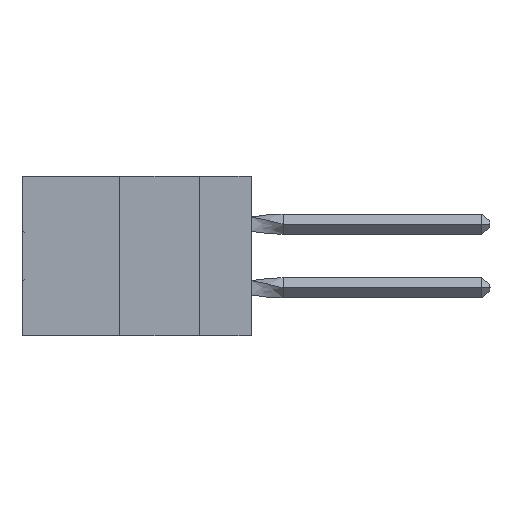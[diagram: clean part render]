
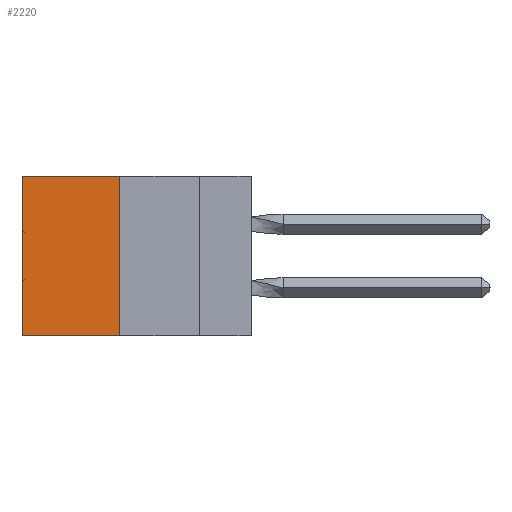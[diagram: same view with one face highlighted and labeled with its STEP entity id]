
A CAD part, left-side view. The second image highlights one B-rep face of the part: STEP entity #2220.
In plain terms, the highlighted planar face has unit normal (-1, 0, 0).
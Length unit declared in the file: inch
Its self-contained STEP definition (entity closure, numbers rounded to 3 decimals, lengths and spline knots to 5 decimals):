
#1751 = ORIENTED_EDGE ( 'NONE', *, *, #40516, .F. ) ;
#1928 = ORIENTED_EDGE ( 'NONE', *, *, #43611, .T. ) ;
#2220 = ADVANCED_FACE ( 'NONE', ( #25682 ), #41466, .F. ) ;
#5457 = LINE ( 'NONE', #10869, #13340 ) ;
#10869 = CARTESIAN_POINT ( 'NONE',  ( 0.305, 0.413, -0.5 ) ) ;
#13340 = VECTOR ( 'NONE', #15083, 39.37008 ) ;
#15083 = DIRECTION ( 'NONE',  ( 0., 1., 0. ) ) ;
#15513 = LINE ( 'NONE', #37387, #19696 ) ;
#15803 = VECTOR ( 'NONE', #25058, 39.37008 ) ;
#17651 = AXIS2_PLACEMENT_3D ( 'NONE', #48975, #22123, #48811 ) ;
#19696 = VECTOR ( 'NONE', #37045, 39.37008 ) ;
#22084 = ORIENTED_EDGE ( 'NONE', *, *, #40361, .T. ) ;
#22123 = DIRECTION ( 'NONE',  ( 1., 0., 0. ) ) ;
#23042 = CARTESIAN_POINT ( 'NONE',  ( 0.305, 0.413, -0.5 ) ) ;
#25058 = DIRECTION ( 'NONE',  ( 0., 1., 0. ) ) ;
#25682 = FACE_OUTER_BOUND ( 'NONE', #30534, .T. ) ;
#26971 = VECTOR ( 'NONE', #47237, 39.37008 ) ;
#27867 = LINE ( 'NONE', #33345, #15803 ) ;
#30534 = EDGE_LOOP ( 'NONE', ( #1928, #1751, #40982, #22084 ) ) ;
#33345 = CARTESIAN_POINT ( 'NONE',  ( 0.305, 0.413, 0. ) ) ;
#33738 = CARTESIAN_POINT ( 'NONE',  ( 0.305, 0.413, 0. ) ) ;
#34742 = EDGE_CURVE ( 'NONE', #38054, #37911, #39719, .T. ) ;
#37045 = DIRECTION ( 'NONE',  ( 0., 0., -1. ) ) ;
#37387 = CARTESIAN_POINT ( 'NONE',  ( 0.305, 0.72, -0.5 ) ) ;
#37911 = VERTEX_POINT ( 'NONE', #23042 ) ;
#38054 = VERTEX_POINT ( 'NONE', #33738 ) ;
#39656 = VERTEX_POINT ( 'NONE', #47721 ) ;
#39719 = LINE ( 'NONE', #44183, #26971 ) ;
#40361 = EDGE_CURVE ( 'NONE', #38054, #41887, #27867, .T. ) ;
#40516 = EDGE_CURVE ( 'NONE', #37911, #39656, #5457, .T. ) ;
#40982 = ORIENTED_EDGE ( 'NONE', *, *, #34742, .F. ) ;
#41466 = PLANE ( 'NONE',  #17651 ) ;
#41887 = VERTEX_POINT ( 'NONE', #47002 ) ;
#43611 = EDGE_CURVE ( 'NONE', #41887, #39656, #15513, .T. ) ;
#44183 = CARTESIAN_POINT ( 'NONE',  ( 0.305, 0.413, -0.5 ) ) ;
#47002 = CARTESIAN_POINT ( 'NONE',  ( 0.305, 0.72, 0. ) ) ;
#47237 = DIRECTION ( 'NONE',  ( 0., 0., -1. ) ) ;
#47721 = CARTESIAN_POINT ( 'NONE',  ( 0.305, 0.72, -0.5 ) ) ;
#48811 = DIRECTION ( 'NONE',  ( 0., 0., -1. ) ) ;
#48975 = CARTESIAN_POINT ( 'NONE',  ( 0.305, 0.413, -0.5 ) ) ;
